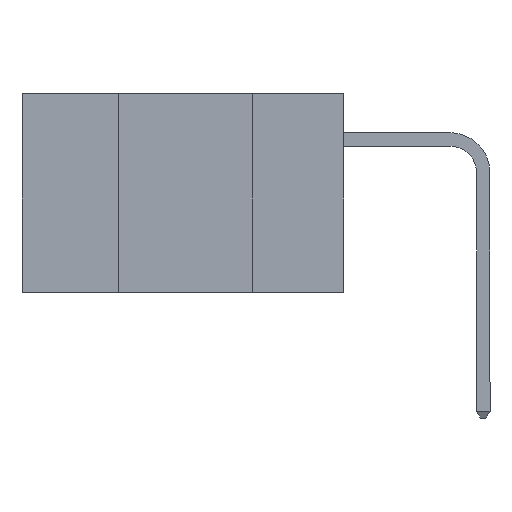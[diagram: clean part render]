
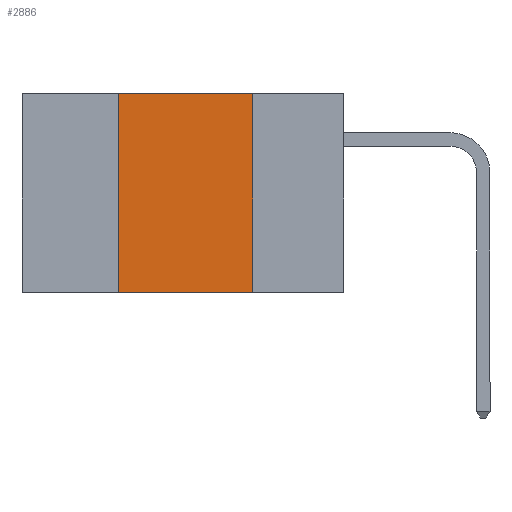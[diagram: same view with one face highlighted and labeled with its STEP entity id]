
A CAD part, left-side view. The second image highlights one B-rep face of the part: STEP entity #2886.
In plain terms, the highlighted planar face has unit normal (-1, 0, 0).
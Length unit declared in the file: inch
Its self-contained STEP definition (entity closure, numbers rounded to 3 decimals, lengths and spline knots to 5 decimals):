
#573 = ORIENTED_EDGE ( 'NONE', *, *, #5754, .F. ) ;
#891 = ORIENTED_EDGE ( 'NONE', *, *, #3870, .F. ) ;
#928 = CARTESIAN_POINT ( 'NONE',  ( 0., 0.42, -0.37 ) ) ;
#1143 = CARTESIAN_POINT ( 'NONE',  ( 0., 0.6, -0.37 ) ) ;
#1587 = VERTEX_POINT ( 'NONE', #1685 ) ;
#1685 = CARTESIAN_POINT ( 'NONE',  ( 0., 0.17, -0.37 ) ) ;
#1848 = VERTEX_POINT ( 'NONE', #928 ) ;
#2330 = VECTOR ( 'NONE', #13550, 39.37008 ) ;
#2527 = CARTESIAN_POINT ( 'NONE',  ( 0., 0.42, 0. ) ) ;
#2886 = ADVANCED_FACE ( 'NONE', ( #5654 ), #3585, .F. ) ;
#3387 = EDGE_CURVE ( 'NONE', #4398, #1587, #5300, .T. ) ;
#3585 = PLANE ( 'NONE',  #9300 ) ;
#3870 = EDGE_CURVE ( 'NONE', #1848, #6164, #12902, .T. ) ;
#4398 = VERTEX_POINT ( 'NONE', #7985 ) ;
#4776 = DIRECTION ( 'NONE',  ( 0., 0., 1. ) ) ;
#4792 = CARTESIAN_POINT ( 'NONE',  ( 0., 0.6, 0. ) ) ;
#5146 = DIRECTION ( 'NONE',  ( 0., -1., 0. ) ) ;
#5300 = LINE ( 'NONE', #13480, #2330 ) ;
#5654 = FACE_OUTER_BOUND ( 'NONE', #10129, .T. ) ;
#5754 = EDGE_CURVE ( 'NONE', #6164, #4398, #11494, .T. ) ;
#5930 = DIRECTION ( 'NONE',  ( 0., 0., -1. ) ) ;
#6155 = CARTESIAN_POINT ( 'NONE',  ( 0., 0.6, 0. ) ) ;
#6164 = VERTEX_POINT ( 'NONE', #6375 ) ;
#6375 = CARTESIAN_POINT ( 'NONE',  ( 0., 0.42, 0. ) ) ;
#6763 = EDGE_CURVE ( 'NONE', #1848, #1587, #9542, .T. ) ;
#6767 = VECTOR ( 'NONE', #8674, 39.37008 ) ;
#7972 = DIRECTION ( 'NONE',  ( 1., 0., 0. ) ) ;
#7985 = CARTESIAN_POINT ( 'NONE',  ( 0., 0.17, 0. ) ) ;
#8058 = VECTOR ( 'NONE', #4776, 39.37008 ) ;
#8405 = VECTOR ( 'NONE', #5146, 39.37008 ) ;
#8477 = ORIENTED_EDGE ( 'NONE', *, *, #3387, .F. ) ;
#8674 = DIRECTION ( 'NONE',  ( 0., -1., 0. ) ) ;
#9300 = AXIS2_PLACEMENT_3D ( 'NONE', #6155, #7972, #5930 ) ;
#9542 = LINE ( 'NONE', #1143, #6767 ) ;
#10129 = EDGE_LOOP ( 'NONE', ( #8477, #573, #891, #11571 ) ) ;
#11494 = LINE ( 'NONE', #4792, #8405 ) ;
#11571 = ORIENTED_EDGE ( 'NONE', *, *, #6763, .T. ) ;
#12902 = LINE ( 'NONE', #2527, #8058 ) ;
#13480 = CARTESIAN_POINT ( 'NONE',  ( 0., 0.17, 0. ) ) ;
#13550 = DIRECTION ( 'NONE',  ( 0., 0., -1. ) ) ;
